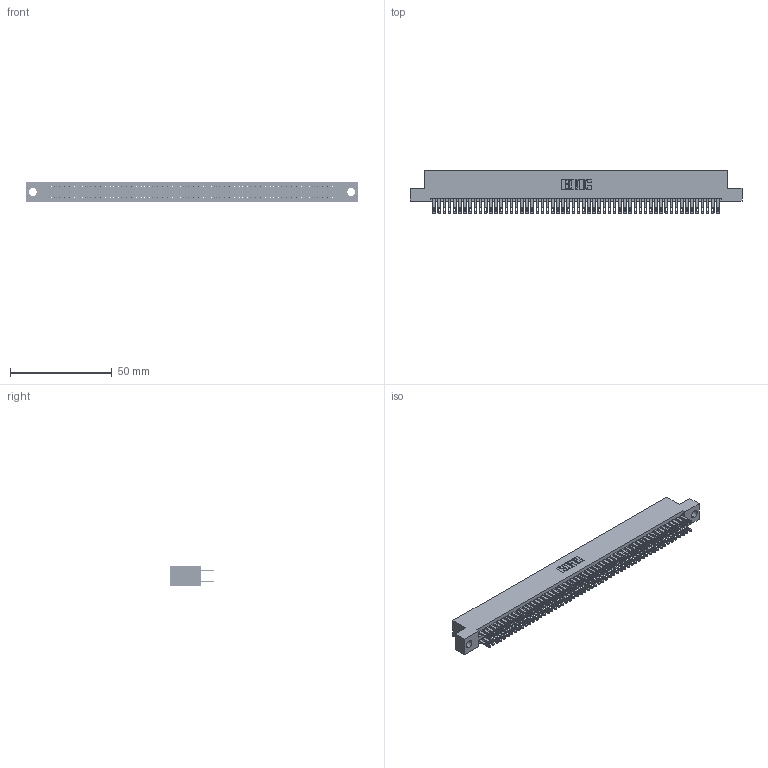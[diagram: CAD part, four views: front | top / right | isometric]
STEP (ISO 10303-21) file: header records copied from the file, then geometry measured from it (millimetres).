
FILE_DESCRIPTION (( 'STEP AP203' ), '1' );
FILE_NAME ('345-112-500-204.STEP', '2021-05-25T14:15:22', ( '' ), ( '' ), 'SwSTEP 2.0', 'SolidWorks 2020', '' );
FILE_SCHEMA (( 'CONFIG_CONTROL_DESIGN' ));
Length unit declared in the file: inch
Products named in the file (3): 345-112-500-204; 345 Part_Flush Mounting Lugs - 0.156 Dia-TI; 345-292-001_345-293-100
Assembly tree (113 placements, depth 2):
  345-112-500-204
    345 Part_Flush Mounting Lugs - 0.156 Dia-TI
    345-292-001_345-293-100  x112
Bounding box: 163.45 x 21.51 x 9.4 mm (x, y, z)
Volume: 16243.9 mm3; surface area: 25276.2 mm2
Topology: 113 solids, 113 shells, 5292 faces, 16169 edges, 10778 vertices
Faces by surface type: plane 3118, cylinder 2174
Entity records: 42403 total; most frequent: CARTESIAN_POINT 7098, ORIENTED_EDGE 7030, DIRECTION 6243, EDGE_CURVE 3515, VECTOR 3155, LINE 3155, VERTEX_POINT 2342, AXIS2_PLACEMENT_3D 1544
